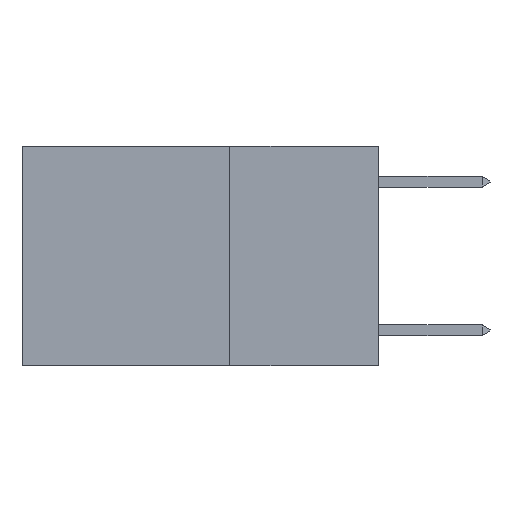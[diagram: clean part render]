
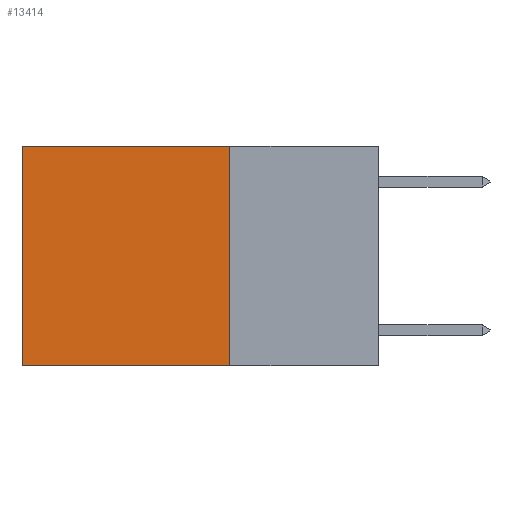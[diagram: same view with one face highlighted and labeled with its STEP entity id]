
A CAD part, left-side view. The second image highlights one B-rep face of the part: STEP entity #13414.
In plain terms, the highlighted planar face has unit normal (-1, 0, 0).
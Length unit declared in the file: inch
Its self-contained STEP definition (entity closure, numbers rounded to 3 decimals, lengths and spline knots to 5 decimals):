
#265 = CARTESIAN_POINT ( 'NONE',  ( 0.2625, 0.25, 0. ) ) ;
#715 = CARTESIAN_POINT ( 'NONE',  ( 0.2625, 0.25, 0. ) ) ;
#880 = VERTEX_POINT ( 'NONE', #6768 ) ;
#1034 = AXIS2_PLACEMENT_3D ( 'NONE', #6042, #15167, #10097 ) ;
#1133 = ORIENTED_EDGE ( 'NONE', *, *, #12488, .F. ) ;
#2822 = DIRECTION ( 'NONE',  ( 0., 1., 0. ) ) ;
#2912 = VERTEX_POINT ( 'NONE', #14617 ) ;
#4340 = LINE ( 'NONE', #4679, #12450 ) ;
#4679 = CARTESIAN_POINT ( 'NONE',  ( 0.2625, 0.25, -0.37 ) ) ;
#6042 = CARTESIAN_POINT ( 'NONE',  ( 0.2625, 0.25, 0. ) ) ;
#6615 = VERTEX_POINT ( 'NONE', #265 ) ;
#6768 = CARTESIAN_POINT ( 'NONE',  ( 0.2625, 0.6, 0. ) ) ;
#6832 = DIRECTION ( 'NONE',  ( 0., 0., -1. ) ) ;
#7323 = VECTOR ( 'NONE', #6832, 39.37008 ) ;
#7750 = ORIENTED_EDGE ( 'NONE', *, *, #12675, .T. ) ;
#8379 = EDGE_CURVE ( 'NONE', #6615, #880, #11769, .T. ) ;
#9207 = CARTESIAN_POINT ( 'NONE',  ( 0.2625, 0.6, 0. ) ) ;
#9311 = VECTOR ( 'NONE', #2822, 39.37008 ) ;
#9491 = DIRECTION ( 'NONE',  ( 0., 1., 0. ) ) ;
#9551 = EDGE_CURVE ( 'NONE', #12092, #2912, #4340, .T. ) ;
#10097 = DIRECTION ( 'NONE',  ( 0., 0., -1. ) ) ;
#10681 = CARTESIAN_POINT ( 'NONE',  ( 0.2625, 0.25, 0. ) ) ;
#10777 = LINE ( 'NONE', #9207, #7323 ) ;
#10883 = ORIENTED_EDGE ( 'NONE', *, *, #8379, .T. ) ;
#11256 = PLANE ( 'NONE',  #1034 ) ;
#11259 = VECTOR ( 'NONE', #13697, 39.37008 ) ;
#11422 = FACE_OUTER_BOUND ( 'NONE', #14495, .T. ) ;
#11769 = LINE ( 'NONE', #10681, #9311 ) ;
#12092 = VERTEX_POINT ( 'NONE', #12341 ) ;
#12304 = ORIENTED_EDGE ( 'NONE', *, *, #9551, .F. ) ;
#12341 = CARTESIAN_POINT ( 'NONE',  ( 0.2625, 0.25, -0.37 ) ) ;
#12450 = VECTOR ( 'NONE', #9491, 39.37008 ) ;
#12488 = EDGE_CURVE ( 'NONE', #6615, #12092, #16206, .T. ) ;
#12675 = EDGE_CURVE ( 'NONE', #880, #2912, #10777, .T. ) ;
#13414 = ADVANCED_FACE ( 'NONE', ( #11422 ), #11256, .F. ) ;
#13697 = DIRECTION ( 'NONE',  ( 0., 0., -1. ) ) ;
#14495 = EDGE_LOOP ( 'NONE', ( #7750, #12304, #1133, #10883 ) ) ;
#14617 = CARTESIAN_POINT ( 'NONE',  ( 0.2625, 0.6, -0.37 ) ) ;
#15167 = DIRECTION ( 'NONE',  ( 1., 0., 0. ) ) ;
#16206 = LINE ( 'NONE', #715, #11259 ) ;
